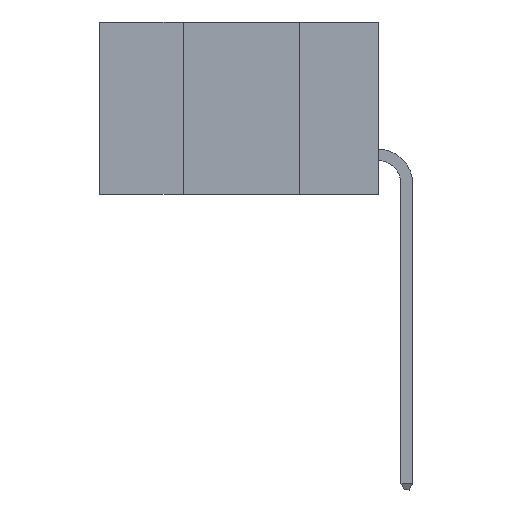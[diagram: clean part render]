
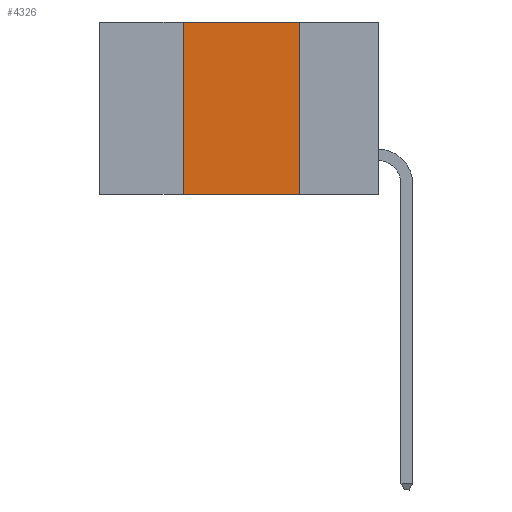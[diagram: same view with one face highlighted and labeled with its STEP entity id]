
A CAD part, left-side view. The second image highlights one B-rep face of the part: STEP entity #4326.
In plain terms, the highlighted planar face has unit normal (-1, 0, 0).
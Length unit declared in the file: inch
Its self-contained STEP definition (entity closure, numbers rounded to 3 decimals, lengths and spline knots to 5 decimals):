
#214 = VECTOR ( 'NONE', #5080, 39.37008 ) ;
#408 = DIRECTION ( 'NONE',  ( 0., 0., -1. ) ) ;
#863 = VECTOR ( 'NONE', #3441, 39.37008 ) ;
#1336 = LINE ( 'NONE', #12847, #12253 ) ;
#3354 = CARTESIAN_POINT ( 'NONE',  ( 0., 0.6, -0.37 ) ) ;
#3441 = DIRECTION ( 'NONE',  ( 0., 0., -1. ) ) ;
#4008 = DIRECTION ( 'NONE',  ( 0., 0., 1. ) ) ;
#4326 = ADVANCED_FACE ( 'NONE', ( #12695 ), #13996, .F. ) ;
#4705 = ORIENTED_EDGE ( 'NONE', *, *, #11128, .F. ) ;
#4922 = CARTESIAN_POINT ( 'NONE',  ( 0., 0.42, -0.37 ) ) ;
#5080 = DIRECTION ( 'NONE',  ( 0., -1., 0. ) ) ;
#5292 = CARTESIAN_POINT ( 'NONE',  ( 0., 0.17, -0.37 ) ) ;
#5313 = CARTESIAN_POINT ( 'NONE',  ( 0., 0.6, 0. ) ) ;
#5479 = LINE ( 'NONE', #14648, #863 ) ;
#6668 = AXIS2_PLACEMENT_3D ( 'NONE', #5313, #15266, #408 ) ;
#7233 = DIRECTION ( 'NONE',  ( 0., -1., 0. ) ) ;
#8396 = LINE ( 'NONE', #3354, #10349 ) ;
#8966 = VERTEX_POINT ( 'NONE', #14809 ) ;
#9858 = VERTEX_POINT ( 'NONE', #11516 ) ;
#9988 = EDGE_CURVE ( 'NONE', #8966, #9858, #15328, .T. ) ;
#10209 = VERTEX_POINT ( 'NONE', #5292 ) ;
#10349 = VECTOR ( 'NONE', #7233, 39.37008 ) ;
#10523 = ORIENTED_EDGE ( 'NONE', *, *, #9988, .F. ) ;
#10952 = VERTEX_POINT ( 'NONE', #4922 ) ;
#11128 = EDGE_CURVE ( 'NONE', #10952, #8966, #1336, .T. ) ;
#11431 = EDGE_LOOP ( 'NONE', ( #12440, #10523, #4705, #15752 ) ) ;
#11516 = CARTESIAN_POINT ( 'NONE',  ( 0., 0.17, 0. ) ) ;
#12253 = VECTOR ( 'NONE', #4008, 39.37008 ) ;
#12440 = ORIENTED_EDGE ( 'NONE', *, *, #12806, .F. ) ;
#12641 = CARTESIAN_POINT ( 'NONE',  ( 0., 0.6, 0. ) ) ;
#12695 = FACE_OUTER_BOUND ( 'NONE', #11431, .T. ) ;
#12806 = EDGE_CURVE ( 'NONE', #9858, #10209, #5479, .T. ) ;
#12847 = CARTESIAN_POINT ( 'NONE',  ( 0., 0.42, 0. ) ) ;
#13996 = PLANE ( 'NONE',  #6668 ) ;
#14356 = EDGE_CURVE ( 'NONE', #10952, #10209, #8396, .T. ) ;
#14648 = CARTESIAN_POINT ( 'NONE',  ( 0., 0.17, 0. ) ) ;
#14809 = CARTESIAN_POINT ( 'NONE',  ( 0., 0.42, 0. ) ) ;
#15266 = DIRECTION ( 'NONE',  ( 1., 0., 0. ) ) ;
#15328 = LINE ( 'NONE', #12641, #214 ) ;
#15752 = ORIENTED_EDGE ( 'NONE', *, *, #14356, .T. ) ;
